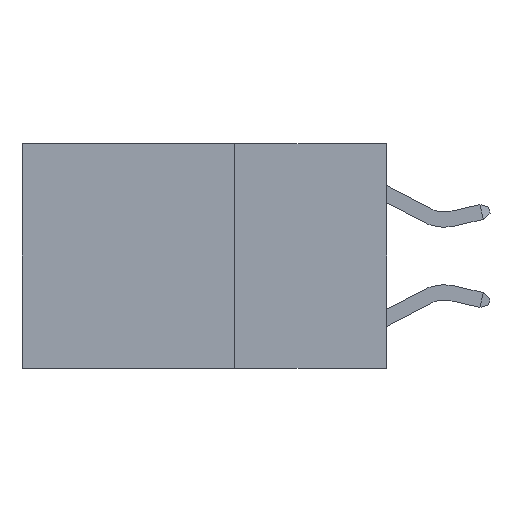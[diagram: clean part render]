
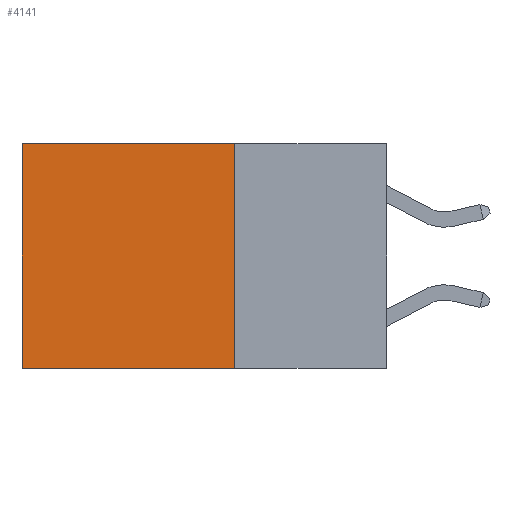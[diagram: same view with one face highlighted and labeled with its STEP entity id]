
A CAD part, left-side view. The second image highlights one B-rep face of the part: STEP entity #4141.
In plain terms, the highlighted planar face has unit normal (-1, 0, 0).
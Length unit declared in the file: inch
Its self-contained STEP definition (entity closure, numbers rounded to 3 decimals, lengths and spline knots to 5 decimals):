
#886 = EDGE_LOOP ( 'NONE', ( #1320, #10639, #3501, #5309 ) ) ;
#909 = PLANE ( 'NONE',  #7644 ) ;
#941 = DIRECTION ( 'NONE',  ( 0., 0., -1. ) ) ;
#957 = VERTEX_POINT ( 'NONE', #1774 ) ;
#997 = DIRECTION ( 'NONE',  ( 0., 1., 0. ) ) ;
#999 = FACE_OUTER_BOUND ( 'NONE', #886, .T. ) ;
#1009 = LINE ( 'NONE', #2032, #10080 ) ;
#1057 = DIRECTION ( 'NONE',  ( 0., 1., 0. ) ) ;
#1320 = ORIENTED_EDGE ( 'NONE', *, *, #3637, .T. ) ;
#1774 = CARTESIAN_POINT ( 'NONE',  ( 0.2625, 0.25, -0.37 ) ) ;
#1894 = CARTESIAN_POINT ( 'NONE',  ( 0.2625, 0.25, -0.37 ) ) ;
#2032 = CARTESIAN_POINT ( 'NONE',  ( 0.2625, 0.6, 0. ) ) ;
#2633 = VERTEX_POINT ( 'NONE', #5363 ) ;
#2635 = DIRECTION ( 'NONE',  ( 1., 0., 0. ) ) ;
#2936 = CARTESIAN_POINT ( 'NONE',  ( 0.2625, 0.25, 0. ) ) ;
#3022 = LINE ( 'NONE', #1894, #7553 ) ;
#3501 = ORIENTED_EDGE ( 'NONE', *, *, #10869, .F. ) ;
#3637 = EDGE_CURVE ( 'NONE', #9224, #2633, #1009, .T. ) ;
#4141 = ADVANCED_FACE ( 'NONE', ( #999 ), #909, .F. ) ;
#4666 = DIRECTION ( 'NONE',  ( 0., 0., -1. ) ) ;
#5309 = ORIENTED_EDGE ( 'NONE', *, *, #6089, .T. ) ;
#5363 = CARTESIAN_POINT ( 'NONE',  ( 0.2625, 0.6, -0.37 ) ) ;
#6089 = EDGE_CURVE ( 'NONE', #9705, #9224, #9875, .T. ) ;
#7412 = LINE ( 'NONE', #7575, #10087 ) ;
#7553 = VECTOR ( 'NONE', #997, 39.37008 ) ;
#7575 = CARTESIAN_POINT ( 'NONE',  ( 0.2625, 0.25, 0. ) ) ;
#7644 = AXIS2_PLACEMENT_3D ( 'NONE', #9312, #2635, #941 ) ;
#8143 = VECTOR ( 'NONE', #1057, 39.37008 ) ;
#9224 = VERTEX_POINT ( 'NONE', #9913 ) ;
#9312 = CARTESIAN_POINT ( 'NONE',  ( 0.2625, 0.25, 0. ) ) ;
#9705 = VERTEX_POINT ( 'NONE', #2936 ) ;
#9875 = LINE ( 'NONE', #10481, #8143 ) ;
#9913 = CARTESIAN_POINT ( 'NONE',  ( 0.2625, 0.6, 0. ) ) ;
#10047 = DIRECTION ( 'NONE',  ( 0., 0., -1. ) ) ;
#10080 = VECTOR ( 'NONE', #4666, 39.37008 ) ;
#10087 = VECTOR ( 'NONE', #10047, 39.37008 ) ;
#10481 = CARTESIAN_POINT ( 'NONE',  ( 0.2625, 0.25, 0. ) ) ;
#10501 = EDGE_CURVE ( 'NONE', #957, #2633, #3022, .T. ) ;
#10639 = ORIENTED_EDGE ( 'NONE', *, *, #10501, .F. ) ;
#10869 = EDGE_CURVE ( 'NONE', #9705, #957, #7412, .T. ) ;
